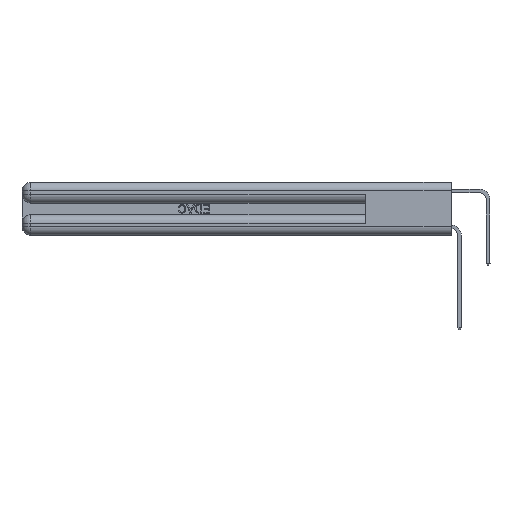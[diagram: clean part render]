
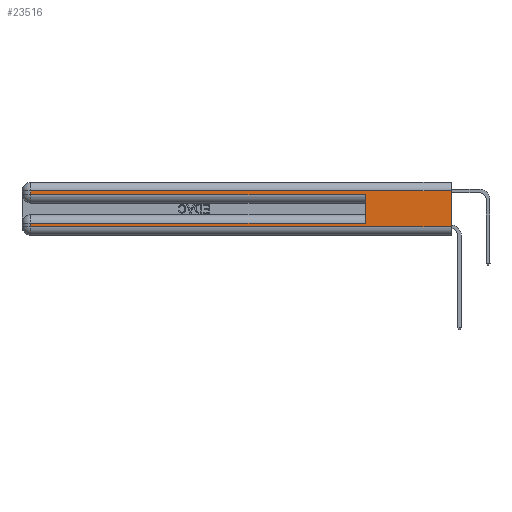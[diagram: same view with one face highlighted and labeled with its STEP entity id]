
A CAD part, left-side view. The second image highlights one B-rep face of the part: STEP entity #23516.
In plain terms, the highlighted planar face has unit normal (-1, 0, 0).
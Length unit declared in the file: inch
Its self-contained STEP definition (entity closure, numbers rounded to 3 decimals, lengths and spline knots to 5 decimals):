
#479 = LINE ( 'NONE', #9064, #35242 ) ;
#1364 = CARTESIAN_POINT ( 'NONE',  ( 0., 0., 0.285 ) ) ;
#1743 = VERTEX_POINT ( 'NONE', #24879 ) ;
#1786 = VECTOR ( 'NONE', #26904, 39.37008 ) ;
#2181 = VERTEX_POINT ( 'NONE', #8753 ) ;
#2574 = CARTESIAN_POINT ( 'NONE',  ( 0., 2.94, 0.37 ) ) ;
#2586 = CARTESIAN_POINT ( 'NONE',  ( 0., 0., 0.085 ) ) ;
#2723 = CARTESIAN_POINT ( 'NONE',  ( 0., 2.94, 0.06 ) ) ;
#2770 = VECTOR ( 'NONE', #21391, 39.37008 ) ;
#2826 = CARTESIAN_POINT ( 'NONE',  ( 0., 0.6, 0.145 ) ) ;
#3023 = AXIS2_PLACEMENT_3D ( 'NONE', #27335, #30208, #30918 ) ;
#3187 = ORIENTED_EDGE ( 'NONE', *, *, #18169, .T. ) ;
#3757 = ORIENTED_EDGE ( 'NONE', *, *, #16742, .T. ) ;
#3828 = VECTOR ( 'NONE', #19387, 39.37008 ) ;
#4660 = EDGE_CURVE ( 'NONE', #6402, #34797, #479, .T. ) ;
#6402 = VERTEX_POINT ( 'NONE', #2723 ) ;
#6748 = CARTESIAN_POINT ( 'NONE',  ( 0., 2.94, 0.285 ) ) ;
#8753 = CARTESIAN_POINT ( 'NONE',  ( 0., 0.6, 0.285 ) ) ;
#9064 = CARTESIAN_POINT ( 'NONE',  ( 0., 0., 0.06 ) ) ;
#10155 = CARTESIAN_POINT ( 'NONE',  ( 0., 0., 0.31 ) ) ;
#11456 = ORIENTED_EDGE ( 'NONE', *, *, #4660, .T. ) ;
#12643 = ORIENTED_EDGE ( 'NONE', *, *, #19725, .T. ) ;
#13184 = VERTEX_POINT ( 'NONE', #13623 ) ;
#13318 = LINE ( 'NONE', #2586, #1786 ) ;
#13623 = CARTESIAN_POINT ( 'NONE',  ( 0., 2.94, 0.085 ) ) ;
#13733 = DIRECTION ( 'NONE',  ( 0., 0., 1. ) ) ;
#14401 = EDGE_CURVE ( 'NONE', #13184, #6402, #22072, .T. ) ;
#14592 = CARTESIAN_POINT ( 'NONE',  ( 0., 0., 0.31 ) ) ;
#14782 = LINE ( 'NONE', #1364, #21772 ) ;
#15857 = LINE ( 'NONE', #10155, #2770 ) ;
#16411 = LINE ( 'NONE', #2826, #34062 ) ;
#16609 = PLANE ( 'NONE',  #3023 ) ;
#16742 = EDGE_CURVE ( 'NONE', #18398, #1743, #15857, .T. ) ;
#16837 = LINE ( 'NONE', #22736, #30941 ) ;
#17114 = CARTESIAN_POINT ( 'NONE',  ( 0., 2.94, 0.37 ) ) ;
#17454 = ORIENTED_EDGE ( 'NONE', *, *, #14401, .T. ) ;
#18169 = EDGE_CURVE ( 'NONE', #1743, #25431, #21936, .T. ) ;
#18398 = VERTEX_POINT ( 'NONE', #14592 ) ;
#18922 = FACE_OUTER_BOUND ( 'NONE', #33427, .T. ) ;
#19387 = DIRECTION ( 'NONE',  ( 0., 0., -1. ) ) ;
#19613 = EDGE_CURVE ( 'NONE', #25431, #2181, #14782, .T. ) ;
#19725 = EDGE_CURVE ( 'NONE', #21123, #13184, #13318, .T. ) ;
#19843 = ORIENTED_EDGE ( 'NONE', *, *, #19613, .T. ) ;
#21123 = VERTEX_POINT ( 'NONE', #26700 ) ;
#21391 = DIRECTION ( 'NONE',  ( 0., 1., 0. ) ) ;
#21772 = VECTOR ( 'NONE', #28543, 39.37008 ) ;
#21936 = LINE ( 'NONE', #17114, #27996 ) ;
#22072 = LINE ( 'NONE', #2574, #3828 ) ;
#22648 = DIRECTION ( 'NONE',  ( 0., -1., 0. ) ) ;
#22736 = CARTESIAN_POINT ( 'NONE',  ( 0., 0., 0.37 ) ) ;
#23516 = ADVANCED_FACE ( 'NONE', ( #18922 ), #16609, .F. ) ;
#24022 = ORIENTED_EDGE ( 'NONE', *, *, #33252, .F. ) ;
#24879 = CARTESIAN_POINT ( 'NONE',  ( 0., 2.94, 0.31 ) ) ;
#25160 = DIRECTION ( 'NONE',  ( 0., 0., -1. ) ) ;
#25407 = DIRECTION ( 'NONE',  ( 0., 0., -1. ) ) ;
#25431 = VERTEX_POINT ( 'NONE', #6748 ) ;
#26700 = CARTESIAN_POINT ( 'NONE',  ( 0., 0.6, 0.085 ) ) ;
#26904 = DIRECTION ( 'NONE',  ( 0., 1., 0. ) ) ;
#26981 = ORIENTED_EDGE ( 'NONE', *, *, #27858, .F. ) ;
#27335 = CARTESIAN_POINT ( 'NONE',  ( 0., 0., 0.37 ) ) ;
#27858 = EDGE_CURVE ( 'NONE', #18398, #34797, #16837, .T. ) ;
#27996 = VECTOR ( 'NONE', #25160, 39.37008 ) ;
#28543 = DIRECTION ( 'NONE',  ( 0., -1., 0. ) ) ;
#30208 = DIRECTION ( 'NONE',  ( 1., 0., 0. ) ) ;
#30918 = DIRECTION ( 'NONE',  ( 0., 0., -1. ) ) ;
#30941 = VECTOR ( 'NONE', #25407, 39.37008 ) ;
#31307 = CARTESIAN_POINT ( 'NONE',  ( 0., 0., 0.06 ) ) ;
#33252 = EDGE_CURVE ( 'NONE', #21123, #2181, #16411, .T. ) ;
#33427 = EDGE_LOOP ( 'NONE', ( #26981, #3757, #3187, #19843, #24022, #12643, #17454, #11456 ) ) ;
#34062 = VECTOR ( 'NONE', #13733, 39.37008 ) ;
#34797 = VERTEX_POINT ( 'NONE', #31307 ) ;
#35242 = VECTOR ( 'NONE', #22648, 39.37008 ) ;
